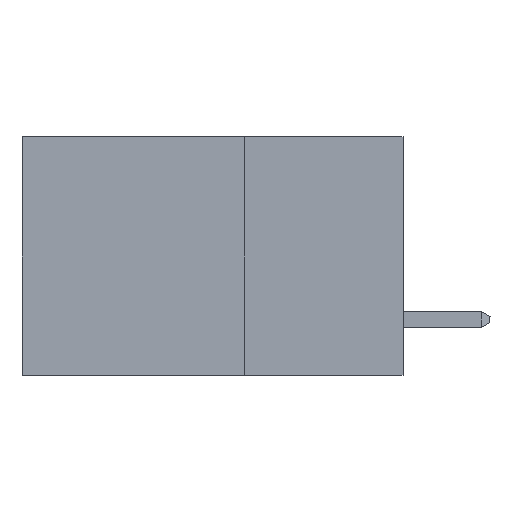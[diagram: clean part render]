
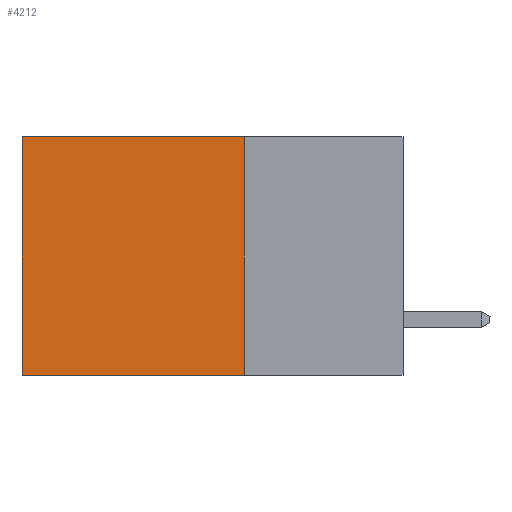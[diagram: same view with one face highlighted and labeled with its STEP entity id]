
A CAD part, left-side view. The second image highlights one B-rep face of the part: STEP entity #4212.
In plain terms, the highlighted planar face has unit normal (-1, 0, 0).
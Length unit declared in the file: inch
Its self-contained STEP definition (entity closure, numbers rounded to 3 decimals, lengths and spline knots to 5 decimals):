
#108 = CARTESIAN_POINT ( 'NONE',  ( 0.2875, 0.6, 0. ) ) ;
#273 = CARTESIAN_POINT ( 'NONE',  ( 0.2875, 0.6, -0.375 ) ) ;
#277 = VERTEX_POINT ( 'NONE', #904 ) ;
#904 = CARTESIAN_POINT ( 'NONE',  ( 0.2875, 0.25, 0. ) ) ;
#1167 = DIRECTION ( 'NONE',  ( 0., 0., -1. ) ) ;
#1219 = VERTEX_POINT ( 'NONE', #273 ) ;
#2265 = LINE ( 'NONE', #4557, #11179 ) ;
#2414 = ORIENTED_EDGE ( 'NONE', *, *, #3003, .F. ) ;
#2626 = ORIENTED_EDGE ( 'NONE', *, *, #5678, .T. ) ;
#3003 = EDGE_CURVE ( 'NONE', #3346, #1219, #7992, .T. ) ;
#3346 = VERTEX_POINT ( 'NONE', #6808 ) ;
#3425 = EDGE_CURVE ( 'NONE', #13608, #1219, #14902, .T. ) ;
#3884 = PLANE ( 'NONE',  #11912 ) ;
#4212 = ADVANCED_FACE ( 'NONE', ( #5199 ), #3884, .F. ) ;
#4557 = CARTESIAN_POINT ( 'NONE',  ( 0.2875, 0.25, 0. ) ) ;
#4574 = CARTESIAN_POINT ( 'NONE',  ( 0.2875, 0.25, -0.375 ) ) ;
#4623 = DIRECTION ( 'NONE',  ( 0., 1., 0. ) ) ;
#5067 = DIRECTION ( 'NONE',  ( 1., 0., 0. ) ) ;
#5117 = DIRECTION ( 'NONE',  ( 0., 0., -1. ) ) ;
#5199 = FACE_OUTER_BOUND ( 'NONE', #5819, .T. ) ;
#5640 = CARTESIAN_POINT ( 'NONE',  ( 0.2875, 0.25, -0.375 ) ) ;
#5678 = EDGE_CURVE ( 'NONE', #277, #13608, #2265, .T. ) ;
#5819 = EDGE_LOOP ( 'NONE', ( #12565, #2414, #6133, #2626 ) ) ;
#6133 = ORIENTED_EDGE ( 'NONE', *, *, #7229, .F. ) ;
#6409 = LINE ( 'NONE', #5640, #10405 ) ;
#6808 = CARTESIAN_POINT ( 'NONE',  ( 0.2875, 0.25, -0.375 ) ) ;
#7229 = EDGE_CURVE ( 'NONE', #277, #3346, #6409, .T. ) ;
#7992 = LINE ( 'NONE', #4574, #8876 ) ;
#7994 = DIRECTION ( 'NONE',  ( 0., 1., 0. ) ) ;
#7998 = DIRECTION ( 'NONE',  ( 0., 0., -1. ) ) ;
#8876 = VECTOR ( 'NONE', #4623, 39.37008 ) ;
#9319 = CARTESIAN_POINT ( 'NONE',  ( 0.2875, 0.6, -0.375 ) ) ;
#9766 = CARTESIAN_POINT ( 'NONE',  ( 0.2875, 0.25, -0.375 ) ) ;
#10405 = VECTOR ( 'NONE', #7998, 39.37008 ) ;
#11179 = VECTOR ( 'NONE', #7994, 39.37008 ) ;
#11912 = AXIS2_PLACEMENT_3D ( 'NONE', #9766, #5067, #5117 ) ;
#12125 = VECTOR ( 'NONE', #1167, 39.37008 ) ;
#12565 = ORIENTED_EDGE ( 'NONE', *, *, #3425, .T. ) ;
#13608 = VERTEX_POINT ( 'NONE', #108 ) ;
#14902 = LINE ( 'NONE', #9319, #12125 ) ;
